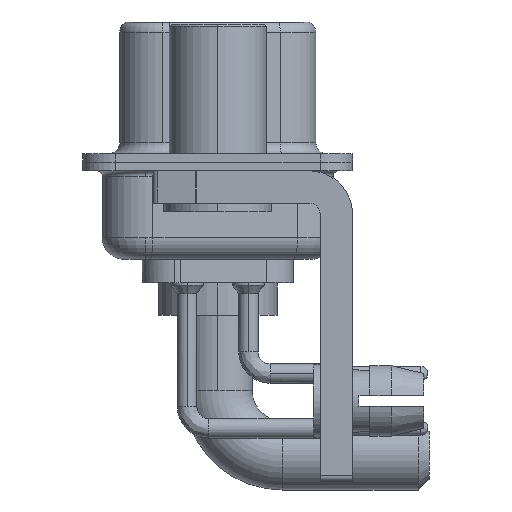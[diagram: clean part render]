
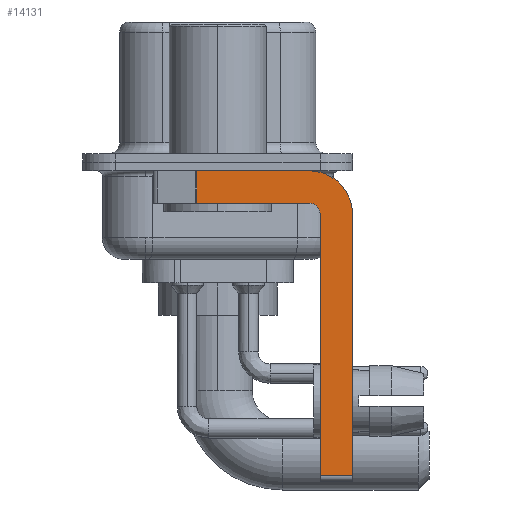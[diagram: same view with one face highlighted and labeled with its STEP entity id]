
A CAD part, left-side view. The second image highlights one B-rep face of the part: STEP entity #14131.
In plain terms, the highlighted planar face has unit normal (-1, 0, 0).
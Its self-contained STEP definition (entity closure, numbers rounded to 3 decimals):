
#1033 = CARTESIAN_POINT ( 'NONE',  ( -2.9, -4.25, -2.4 ) ) ;
#2131 = AXIS2_PLACEMENT_3D ( 'NONE', #1033, #24755, #12573 ) ;
#2379 = CARTESIAN_POINT ( 'NONE',  ( -2.9, -4.25, -1.9 ) ) ;
#2680 = CARTESIAN_POINT ( 'NONE',  ( -2.9, -4.25, -0.4 ) ) ;
#2853 = CARTESIAN_POINT ( 'NONE',  ( -2.9, 0.978, -1.9 ) ) ;
#3443 = EDGE_LOOP ( 'NONE', ( #7909, #8514, #4601, #14152, #17201, #23327, #4001, #15893 ) ) ;
#4001 = ORIENTED_EDGE ( 'NONE', *, *, #11564, .F. ) ;
#4176 = VECTOR ( 'NONE', #10506, 1000. ) ;
#4601 = ORIENTED_EDGE ( 'NONE', *, *, #5785, .F. ) ;
#5202 = DIRECTION ( 'NONE',  ( 0., 0., -1. ) ) ;
#5785 = EDGE_CURVE ( 'NONE', #25474, #18997, #6322, .T. ) ;
#5883 = CARTESIAN_POINT ( 'NONE',  ( -2.9, -6.25, -2.4 ) ) ;
#6270 = DIRECTION ( 'NONE',  ( 0., 0., 1. ) ) ;
#6322 = LINE ( 'NONE', #2379, #4176 ) ;
#6980 = AXIS2_PLACEMENT_3D ( 'NONE', #13013, #17216, #25055 ) ;
#7572 = DIRECTION ( 'NONE',  ( 0., 0., -1. ) ) ;
#7593 = VECTOR ( 'NONE', #12532, 1000. ) ;
#7647 = AXIS2_PLACEMENT_3D ( 'NONE', #22894, #7773, #5202 ) ;
#7773 = DIRECTION ( 'NONE',  ( 1., 0., 0. ) ) ;
#7909 = ORIENTED_EDGE ( 'NONE', *, *, #21940, .F. ) ;
#8072 = CARTESIAN_POINT ( 'NONE',  ( -2.9, -6.25, -14.55 ) ) ;
#8514 = ORIENTED_EDGE ( 'NONE', *, *, #10686, .T. ) ;
#8778 = FACE_OUTER_BOUND ( 'NONE', #3443, .T. ) ;
#8798 = LINE ( 'NONE', #16668, #22431 ) ;
#10194 = CARTESIAN_POINT ( 'NONE',  ( -2.9, 0.978, -0.4 ) ) ;
#10198 = LINE ( 'NONE', #20047, #21028 ) ;
#10488 = PLANE ( 'NONE',  #2131 ) ;
#10506 = DIRECTION ( 'NONE',  ( 0., 1., 0. ) ) ;
#10686 = EDGE_CURVE ( 'NONE', #11702, #18997, #24585, .T. ) ;
#11564 = EDGE_CURVE ( 'NONE', #12582, #19188, #23312, .T. ) ;
#11702 = VERTEX_POINT ( 'NONE', #10194 ) ;
#11951 = EDGE_CURVE ( 'NONE', #15054, #12582, #17716, .T. ) ;
#12532 = DIRECTION ( 'NONE',  ( 0., 0., -1. ) ) ;
#12573 = DIRECTION ( 'NONE',  ( 0., 0., -1. ) ) ;
#12582 = VERTEX_POINT ( 'NONE', #5883 ) ;
#12631 = EDGE_CURVE ( 'NONE', #19185, #20158, #10198, .T. ) ;
#13013 = CARTESIAN_POINT ( 'NONE',  ( -2.9, -4.25, -2.4 ) ) ;
#14131 = ADVANCED_FACE ( 'NONE', ( #8778 ), #10488, .F. ) ;
#14152 = ORIENTED_EDGE ( 'NONE', *, *, #18129, .F. ) ;
#15054 = VERTEX_POINT ( 'NONE', #2680 ) ;
#15746 = CARTESIAN_POINT ( 'NONE',  ( -2.9, 0.978, -1.9 ) ) ;
#15893 = ORIENTED_EDGE ( 'NONE', *, *, #11951, .F. ) ;
#15947 = CARTESIAN_POINT ( 'NONE',  ( -2.9, -4.75, -14.55 ) ) ;
#16496 = CARTESIAN_POINT ( 'NONE',  ( -2.9, -4.75, -2.4 ) ) ;
#16668 = CARTESIAN_POINT ( 'NONE',  ( -2.9, 3., -0.4 ) ) ;
#17201 = ORIENTED_EDGE ( 'NONE', *, *, #12631, .F. ) ;
#17216 = DIRECTION ( 'NONE',  ( -1., 0., 0. ) ) ;
#17461 = CIRCLE ( 'NONE', #6980, 0.5 ) ;
#17716 = CIRCLE ( 'NONE', #7647, 2. ) ;
#18129 = EDGE_CURVE ( 'NONE', #20158, #25474, #17461, .T. ) ;
#18569 = EDGE_CURVE ( 'NONE', #19185, #19188, #21235, .T. ) ;
#18997 = VERTEX_POINT ( 'NONE', #2853 ) ;
#19185 = VERTEX_POINT ( 'NONE', #15947 ) ;
#19188 = VERTEX_POINT ( 'NONE', #8072 ) ;
#20047 = CARTESIAN_POINT ( 'NONE',  ( -2.9, -4.75, -14.8 ) ) ;
#20158 = VERTEX_POINT ( 'NONE', #16496 ) ;
#20221 = VECTOR ( 'NONE', #7572, 1000. ) ;
#20717 = DIRECTION ( 'NONE',  ( 0., -1., 0. ) ) ;
#21028 = VECTOR ( 'NONE', #6270, 1000. ) ;
#21235 = LINE ( 'NONE', #22929, #25322 ) ;
#21732 = CARTESIAN_POINT ( 'NONE',  ( -2.9, -4.25, -1.9 ) ) ;
#21940 = EDGE_CURVE ( 'NONE', #11702, #15054, #8798, .T. ) ;
#22431 = VECTOR ( 'NONE', #24650, 1000. ) ;
#22894 = CARTESIAN_POINT ( 'NONE',  ( -2.9, -4.25, -2.4 ) ) ;
#22929 = CARTESIAN_POINT ( 'NONE',  ( -2.9, -4.25, -14.55 ) ) ;
#23312 = LINE ( 'NONE', #25395, #20221 ) ;
#23327 = ORIENTED_EDGE ( 'NONE', *, *, #18569, .T. ) ;
#24585 = LINE ( 'NONE', #15746, #7593 ) ;
#24650 = DIRECTION ( 'NONE',  ( 0., -1., 0. ) ) ;
#24755 = DIRECTION ( 'NONE',  ( 1., 0., 0. ) ) ;
#25055 = DIRECTION ( 'NONE',  ( 0., 0., 1. ) ) ;
#25322 = VECTOR ( 'NONE', #20717, 1000. ) ;
#25395 = CARTESIAN_POINT ( 'NONE',  ( -2.9, -6.25, -2.4 ) ) ;
#25474 = VERTEX_POINT ( 'NONE', #21732 ) ;
